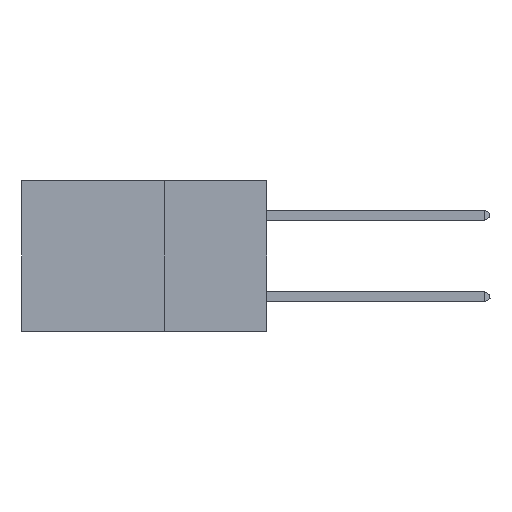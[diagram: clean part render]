
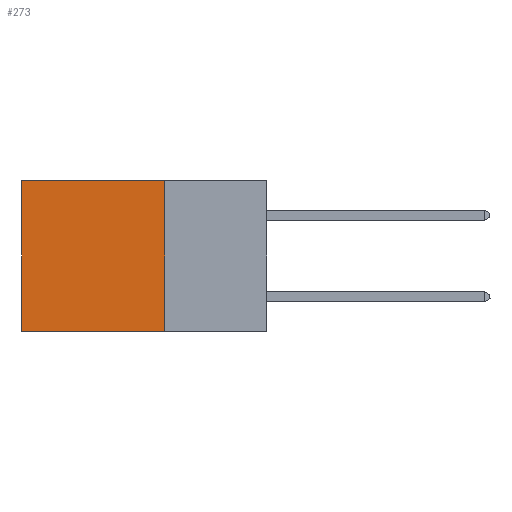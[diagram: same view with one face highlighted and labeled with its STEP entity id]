
A CAD part, left-side view. The second image highlights one B-rep face of the part: STEP entity #273.
In plain terms, the highlighted planar face has unit normal (-1, 0, 0).
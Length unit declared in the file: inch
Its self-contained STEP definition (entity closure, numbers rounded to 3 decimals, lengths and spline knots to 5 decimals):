
#164 = EDGE_CURVE ( 'NONE', #1632, #10380, #6886, .T. ) ;
#273 = ADVANCED_FACE ( 'NONE', ( #4985 ), #14004, .F. ) ;
#706 = CARTESIAN_POINT ( 'NONE',  ( 0.2875, 0.25, 0. ) ) ;
#960 = VECTOR ( 'NONE', #1684, 39.37008 ) ;
#1030 = VECTOR ( 'NONE', #2723, 39.37008 ) ;
#1632 = VERTEX_POINT ( 'NONE', #8576 ) ;
#1684 = DIRECTION ( 'NONE',  ( 0., 1., 0. ) ) ;
#2185 = DIRECTION ( 'NONE',  ( 0., 0., -1. ) ) ;
#2723 = DIRECTION ( 'NONE',  ( 0., 1., 0. ) ) ;
#2795 = LINE ( 'NONE', #9051, #960 ) ;
#4985 = FACE_OUTER_BOUND ( 'NONE', #6430, .T. ) ;
#5369 = CARTESIAN_POINT ( 'NONE',  ( 0.2875, 0.25, 0. ) ) ;
#5546 = DIRECTION ( 'NONE',  ( 1., 0., 0. ) ) ;
#5853 = DIRECTION ( 'NONE',  ( 0., 0., -1. ) ) ;
#5889 = AXIS2_PLACEMENT_3D ( 'NONE', #5369, #5546, #13215 ) ;
#6345 = EDGE_CURVE ( 'NONE', #16853, #15223, #16409, .T. ) ;
#6430 = EDGE_LOOP ( 'NONE', ( #11361, #18121, #8788, #18326 ) ) ;
#6503 = CARTESIAN_POINT ( 'NONE',  ( 0.2875, 0.6, 0. ) ) ;
#6886 = LINE ( 'NONE', #706, #14067 ) ;
#8576 = CARTESIAN_POINT ( 'NONE',  ( 0.2875, 0.25, 0. ) ) ;
#8788 = ORIENTED_EDGE ( 'NONE', *, *, #164, .F. ) ;
#9051 = CARTESIAN_POINT ( 'NONE',  ( 0.2875, 0.25, 0. ) ) ;
#9325 = LINE ( 'NONE', #15771, #1030 ) ;
#10380 = VERTEX_POINT ( 'NONE', #17756 ) ;
#11361 = ORIENTED_EDGE ( 'NONE', *, *, #6345, .T. ) ;
#13077 = VECTOR ( 'NONE', #5853, 39.37008 ) ;
#13215 = DIRECTION ( 'NONE',  ( 0., 0., -1. ) ) ;
#13505 = EDGE_CURVE ( 'NONE', #10380, #15223, #9325, .T. ) ;
#13934 = CARTESIAN_POINT ( 'NONE',  ( 0.2875, 0.6, -0.37 ) ) ;
#14004 = PLANE ( 'NONE',  #5889 ) ;
#14067 = VECTOR ( 'NONE', #2185, 39.37008 ) ;
#15223 = VERTEX_POINT ( 'NONE', #13934 ) ;
#15771 = CARTESIAN_POINT ( 'NONE',  ( 0.2875, 0.25, -0.37 ) ) ;
#16409 = LINE ( 'NONE', #16920, #13077 ) ;
#16639 = EDGE_CURVE ( 'NONE', #1632, #16853, #2795, .T. ) ;
#16853 = VERTEX_POINT ( 'NONE', #6503 ) ;
#16920 = CARTESIAN_POINT ( 'NONE',  ( 0.2875, 0.6, 0. ) ) ;
#17756 = CARTESIAN_POINT ( 'NONE',  ( 0.2875, 0.25, -0.37 ) ) ;
#18121 = ORIENTED_EDGE ( 'NONE', *, *, #13505, .F. ) ;
#18326 = ORIENTED_EDGE ( 'NONE', *, *, #16639, .T. ) ;
